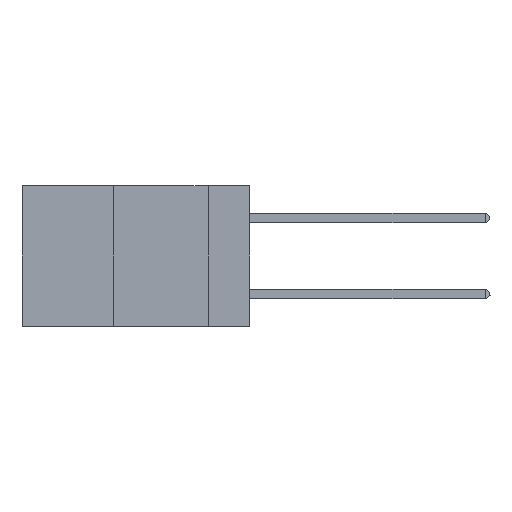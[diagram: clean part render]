
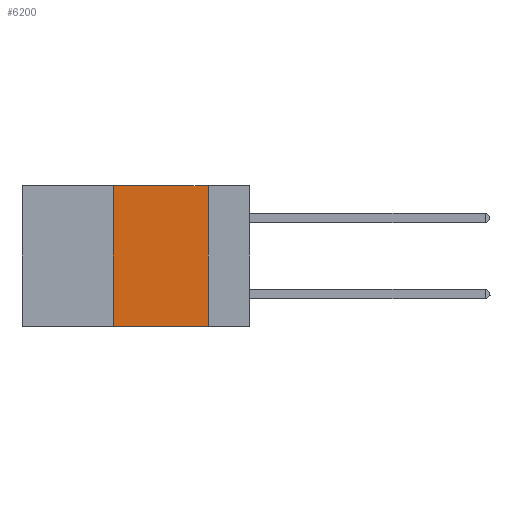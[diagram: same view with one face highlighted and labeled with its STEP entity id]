
A CAD part, left-side view. The second image highlights one B-rep face of the part: STEP entity #6200.
In plain terms, the highlighted planar face has unit normal (-1, 0, 0).
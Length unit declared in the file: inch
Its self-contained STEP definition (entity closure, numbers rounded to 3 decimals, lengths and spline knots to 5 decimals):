
#1539 = DIRECTION ( 'NONE',  ( 0., 0., 1. ) ) ;
#3679 = LINE ( 'NONE', #20974, #19771 ) ;
#4064 = DIRECTION ( 'NONE',  ( 0., -1., 0. ) ) ;
#4367 = ORIENTED_EDGE ( 'NONE', *, *, #17802, .F. ) ;
#4573 = CARTESIAN_POINT ( 'NONE',  ( 0., 0.11, 0. ) ) ;
#4694 = VERTEX_POINT ( 'NONE', #4573 ) ;
#5408 = VERTEX_POINT ( 'NONE', #15184 ) ;
#6200 = ADVANCED_FACE ( 'NONE', ( #16893 ), #23095, .F. ) ;
#6214 = DIRECTION ( 'NONE',  ( 0., 0., -1. ) ) ;
#6309 = DIRECTION ( 'NONE',  ( 1., 0., 0. ) ) ;
#6890 = ORIENTED_EDGE ( 'NONE', *, *, #16836, .F. ) ;
#9265 = VECTOR ( 'NONE', #4064, 39.37008 ) ;
#9538 = VECTOR ( 'NONE', #1539, 39.37008 ) ;
#10301 = CARTESIAN_POINT ( 'NONE',  ( 0., 0.6, -0.37 ) ) ;
#10403 = LINE ( 'NONE', #10301, #13028 ) ;
#11773 = AXIS2_PLACEMENT_3D ( 'NONE', #18781, #6309, #6214 ) ;
#12133 = CARTESIAN_POINT ( 'NONE',  ( 0., 0.36, 0. ) ) ;
#12328 = DIRECTION ( 'NONE',  ( 0., -1., 0. ) ) ;
#13028 = VECTOR ( 'NONE', #12328, 39.37008 ) ;
#13250 = ORIENTED_EDGE ( 'NONE', *, *, #22809, .T. ) ;
#14591 = DIRECTION ( 'NONE',  ( 0., 0., -1. ) ) ;
#14806 = VERTEX_POINT ( 'NONE', #15415 ) ;
#15184 = CARTESIAN_POINT ( 'NONE',  ( 0., 0.36, 0. ) ) ;
#15415 = CARTESIAN_POINT ( 'NONE',  ( 0., 0.36, -0.37 ) ) ;
#16475 = LINE ( 'NONE', #12133, #9538 ) ;
#16831 = EDGE_CURVE ( 'NONE', #5408, #4694, #20425, .T. ) ;
#16836 = EDGE_CURVE ( 'NONE', #4694, #20760, #3679, .T. ) ;
#16893 = FACE_OUTER_BOUND ( 'NONE', #24563, .T. ) ;
#17054 = CARTESIAN_POINT ( 'NONE',  ( 0., 0.6, 0. ) ) ;
#17802 = EDGE_CURVE ( 'NONE', #14806, #5408, #16475, .T. ) ;
#18781 = CARTESIAN_POINT ( 'NONE',  ( 0., 0.6, 0. ) ) ;
#19771 = VECTOR ( 'NONE', #14591, 39.37008 ) ;
#20425 = LINE ( 'NONE', #17054, #9265 ) ;
#20760 = VERTEX_POINT ( 'NONE', #26475 ) ;
#20974 = CARTESIAN_POINT ( 'NONE',  ( 0., 0.11, 0. ) ) ;
#22809 = EDGE_CURVE ( 'NONE', #14806, #20760, #10403, .T. ) ;
#23095 = PLANE ( 'NONE',  #11773 ) ;
#23703 = ORIENTED_EDGE ( 'NONE', *, *, #16831, .F. ) ;
#24563 = EDGE_LOOP ( 'NONE', ( #6890, #23703, #4367, #13250 ) ) ;
#26475 = CARTESIAN_POINT ( 'NONE',  ( 0., 0.11, -0.37 ) ) ;
